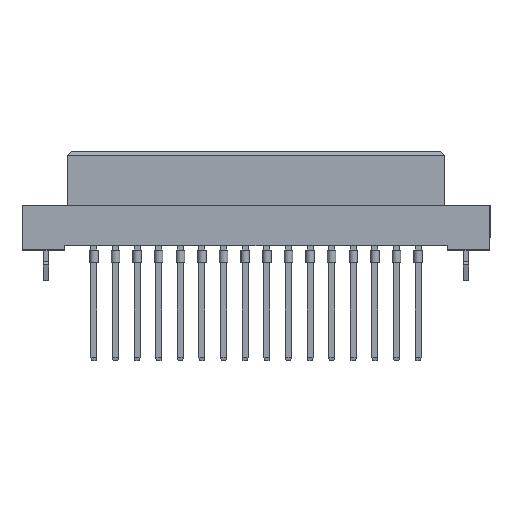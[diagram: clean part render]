
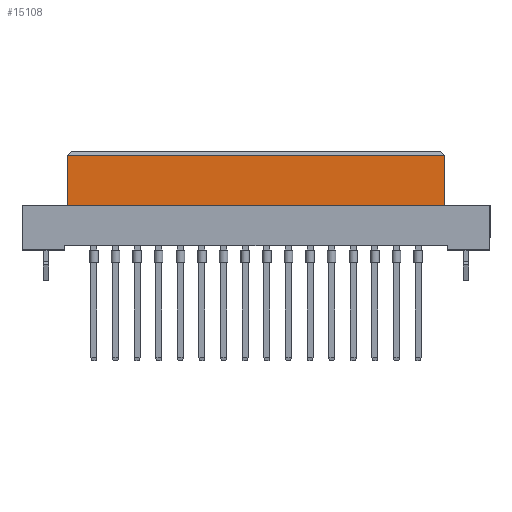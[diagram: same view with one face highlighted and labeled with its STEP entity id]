
A CAD part, top view. The second image highlights one B-rep face of the part: STEP entity #15108.
In plain terms, the highlighted planar face has unit normal (0, 0, 1).
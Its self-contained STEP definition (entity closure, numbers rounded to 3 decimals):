
#308 = EDGE_CURVE ( 'NONE', #21339, #9119, #1366, .T. ) ;
#903 = LINE ( 'NONE', #4635, #8043 ) ;
#1366 = LINE ( 'NONE', #13374, #12710 ) ;
#2033 = VECTOR ( 'NONE', #19564, 1000. ) ;
#2388 = FACE_OUTER_BOUND ( 'NONE', #19309, .T. ) ;
#2605 = DIRECTION ( 'NONE',  ( 1., 0., 0. ) ) ;
#2879 = DIRECTION ( 'NONE',  ( -1., 0., 0. ) ) ;
#3198 = EDGE_CURVE ( 'NONE', #13594, #7910, #11920, .T. ) ;
#3542 = CARTESIAN_POINT ( 'NONE',  ( 22.2, -6.4, 4.25 ) ) ;
#4635 = CARTESIAN_POINT ( 'NONE',  ( -22.2, -0.5, 4.25 ) ) ;
#4805 = ORIENTED_EDGE ( 'NONE', *, *, #11072, .T. ) ;
#4857 = EDGE_CURVE ( 'NONE', #9119, #7910, #903, .T. ) ;
#6016 = DIRECTION ( 'NONE',  ( 0., 0., 1. ) ) ;
#6569 = ORIENTED_EDGE ( 'NONE', *, *, #4857, .T. ) ;
#6855 = CARTESIAN_POINT ( 'NONE',  ( -22.2, -6.4, 4.25 ) ) ;
#7910 = VERTEX_POINT ( 'NONE', #10177 ) ;
#8043 = VECTOR ( 'NONE', #2879, 1000. ) ;
#8136 = ORIENTED_EDGE ( 'NONE', *, *, #3198, .F. ) ;
#8307 = DIRECTION ( 'NONE',  ( 0., 1., 0. ) ) ;
#8329 = VECTOR ( 'NONE', #8307, 1000. ) ;
#9111 = PLANE ( 'NONE',  #12477 ) ;
#9119 = VERTEX_POINT ( 'NONE', #12707 ) ;
#10177 = CARTESIAN_POINT ( 'NONE',  ( -22.2, -0.5, 4.25 ) ) ;
#11072 = EDGE_CURVE ( 'NONE', #13594, #21339, #15744, .T. ) ;
#11920 = LINE ( 'NONE', #6855, #8329 ) ;
#12477 = AXIS2_PLACEMENT_3D ( 'NONE', #14484, #6016, #2605 ) ;
#12707 = CARTESIAN_POINT ( 'NONE',  ( 22.2, -0.5, 4.25 ) ) ;
#12710 = VECTOR ( 'NONE', #18189, 1000. ) ;
#13085 = CARTESIAN_POINT ( 'NONE',  ( -22.2, -6.4, 4.25 ) ) ;
#13374 = CARTESIAN_POINT ( 'NONE',  ( 22.2, -6.4, 4.25 ) ) ;
#13594 = VERTEX_POINT ( 'NONE', #13085 ) ;
#14205 = CARTESIAN_POINT ( 'NONE',  ( 22.2, -6.4, 4.25 ) ) ;
#14484 = CARTESIAN_POINT ( 'NONE',  ( 22.2, -6.4, 4.25 ) ) ;
#15108 = ADVANCED_FACE ( 'NONE', ( #2388 ), #9111, .T. ) ;
#15744 = LINE ( 'NONE', #14205, #2033 ) ;
#18189 = DIRECTION ( 'NONE',  ( 0., 1., 0. ) ) ;
#18477 = ORIENTED_EDGE ( 'NONE', *, *, #308, .T. ) ;
#19309 = EDGE_LOOP ( 'NONE', ( #18477, #6569, #8136, #4805 ) ) ;
#19564 = DIRECTION ( 'NONE',  ( 1., 0., 0. ) ) ;
#21339 = VERTEX_POINT ( 'NONE', #3542 ) ;
